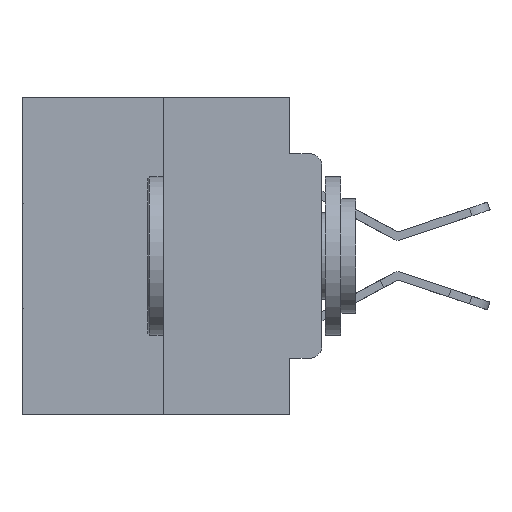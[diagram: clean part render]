
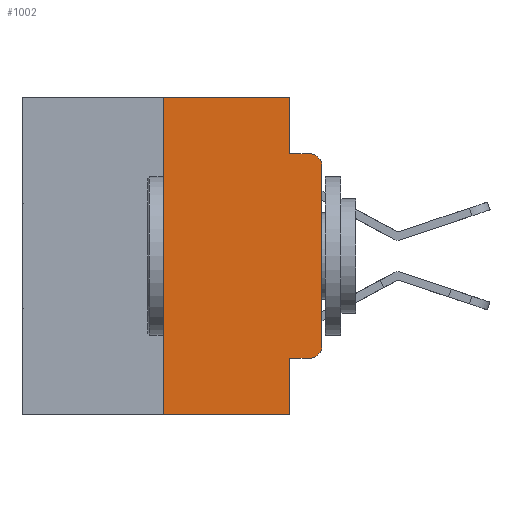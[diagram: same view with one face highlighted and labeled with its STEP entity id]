
A CAD part, left-side view. The second image highlights one B-rep face of the part: STEP entity #1002.
In plain terms, the highlighted planar face has unit normal (-1, 0, 0).
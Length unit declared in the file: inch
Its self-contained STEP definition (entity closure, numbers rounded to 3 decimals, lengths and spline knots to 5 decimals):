
#64 = CIRCLE ( 'NONE', #6986, 0.02 ) ;
#742 = DIRECTION ( 'NONE',  ( 0., -1., 0. ) ) ;
#959 = EDGE_CURVE ( 'NONE', #15801, #18309, #8363, .T. ) ;
#1002 = ADVANCED_FACE ( 'NONE', ( #3110 ), #13808, .F. ) ;
#1123 = DIRECTION ( 'NONE',  ( 0., 0., 1. ) ) ;
#1783 = CARTESIAN_POINT ( 'NONE',  ( 0., 0.473, 0. ) ) ;
#2193 = CARTESIAN_POINT ( 'NONE',  ( 0., 0.051, -0.4115 ) ) ;
#2379 = CIRCLE ( 'NONE', #25160, 0.02 ) ;
#3077 = ORIENTED_EDGE ( 'NONE', *, *, #23673, .F. ) ;
#3110 = FACE_OUTER_BOUND ( 'NONE', #18369, .T. ) ;
#3456 = LINE ( 'NONE', #24547, #14738 ) ;
#4176 = LINE ( 'NONE', #27578, #14776 ) ;
#4309 = AXIS2_PLACEMENT_3D ( 'NONE', #1783, #17391, #17080 ) ;
#4552 = VERTEX_POINT ( 'NONE', #12785 ) ;
#4573 = EDGE_CURVE ( 'NONE', #16203, #19289, #7102, .T. ) ;
#4838 = LINE ( 'NONE', #7823, #10851 ) ;
#6986 = AXIS2_PLACEMENT_3D ( 'NONE', #11329, #27059, #13607 ) ;
#7102 = LINE ( 'NONE', #12881, #24487 ) ;
#7797 = VECTOR ( 'NONE', #16236, 39.37008 ) ;
#7823 = CARTESIAN_POINT ( 'NONE',  ( 0., 0.051, 0. ) ) ;
#8363 = LINE ( 'NONE', #16173, #13659 ) ;
#8471 = VERTEX_POINT ( 'NONE', #2193 ) ;
#8494 = CARTESIAN_POINT ( 'NONE',  ( 0., 0.051, 0. ) ) ;
#8728 = ORIENTED_EDGE ( 'NONE', *, *, #24526, .F. ) ;
#9481 = VERTEX_POINT ( 'NONE', #17270 ) ;
#9647 = CARTESIAN_POINT ( 'NONE',  ( 0., 0.473, -0.5 ) ) ;
#10197 = CARTESIAN_POINT ( 'NONE',  ( 0., 0.25, -0.5 ) ) ;
#10491 = ORIENTED_EDGE ( 'NONE', *, *, #27255, .F. ) ;
#10586 = DIRECTION ( 'NONE',  ( 0., 0., 1. ) ) ;
#10818 = CARTESIAN_POINT ( 'NONE',  ( 0., 0.051, 0. ) ) ;
#10851 = VECTOR ( 'NONE', #12382, 39.37008 ) ;
#10988 = EDGE_CURVE ( 'NONE', #8471, #4552, #13813, .T. ) ;
#11183 = CARTESIAN_POINT ( 'NONE',  ( 0., 0., -0.1085 ) ) ;
#11329 = CARTESIAN_POINT ( 'NONE',  ( 0., 0.02, -0.3915 ) ) ;
#11498 = LINE ( 'NONE', #8494, #16125 ) ;
#11652 = VERTEX_POINT ( 'NONE', #25169 ) ;
#11654 = CARTESIAN_POINT ( 'NONE',  ( 0., 0.051, -0.4115 ) ) ;
#11881 = DIRECTION ( 'NONE',  ( 0., -1., 0. ) ) ;
#12382 = DIRECTION ( 'NONE',  ( 0., 0., -1. ) ) ;
#12596 = ORIENTED_EDGE ( 'NONE', *, *, #17511, .T. ) ;
#12601 = CARTESIAN_POINT ( 'NONE',  ( 0., 0.02, -0.1085 ) ) ;
#12785 = CARTESIAN_POINT ( 'NONE',  ( 0., 0.02, -0.4115 ) ) ;
#12881 = CARTESIAN_POINT ( 'NONE',  ( 0., 0., 0. ) ) ;
#13041 = DIRECTION ( 'NONE',  ( 0., 0., -1. ) ) ;
#13262 = EDGE_CURVE ( 'NONE', #19289, #26048, #2379, .T. ) ;
#13351 = ORIENTED_EDGE ( 'NONE', *, *, #13262, .T. ) ;
#13607 = DIRECTION ( 'NONE',  ( 0., 0., -1. ) ) ;
#13659 = VECTOR ( 'NONE', #1123, 39.37008 ) ;
#13808 = PLANE ( 'NONE',  #4309 ) ;
#13813 = LINE ( 'NONE', #11654, #7797 ) ;
#13824 = CARTESIAN_POINT ( 'NONE',  ( 0., 0., -0.3915 ) ) ;
#14233 = CARTESIAN_POINT ( 'NONE',  ( 0., 0.02, -0.0885 ) ) ;
#14548 = CARTESIAN_POINT ( 'NONE',  ( 0., 0.25, 0. ) ) ;
#14738 = VECTOR ( 'NONE', #26820, 39.37008 ) ;
#14776 = VECTOR ( 'NONE', #11881, 39.37008 ) ;
#14888 = DIRECTION ( 'NONE',  ( 0., 0., -1. ) ) ;
#15801 = VERTEX_POINT ( 'NONE', #10197 ) ;
#16125 = VECTOR ( 'NONE', #13041, 39.37008 ) ;
#16173 = CARTESIAN_POINT ( 'NONE',  ( 0., 0.25, 0. ) ) ;
#16203 = VERTEX_POINT ( 'NONE', #13824 ) ;
#16236 = DIRECTION ( 'NONE',  ( 0., -1., 0. ) ) ;
#17080 = DIRECTION ( 'NONE',  ( 0., 0., -1. ) ) ;
#17270 = CARTESIAN_POINT ( 'NONE',  ( 0., 0.051, -0.5 ) ) ;
#17391 = DIRECTION ( 'NONE',  ( 1., 0., 0. ) ) ;
#17511 = EDGE_CURVE ( 'NONE', #15801, #9481, #26097, .T. ) ;
#18309 = VERTEX_POINT ( 'NONE', #14548 ) ;
#18369 = EDGE_LOOP ( 'NONE', ( #18959, #13351, #25698, #8728, #10491, #28712, #12596, #3077, #18605, #27938 ) ) ;
#18605 = ORIENTED_EDGE ( 'NONE', *, *, #10988, .T. ) ;
#18756 = VECTOR ( 'NONE', #742, 39.37008 ) ;
#18959 = ORIENTED_EDGE ( 'NONE', *, *, #4573, .T. ) ;
#19289 = VERTEX_POINT ( 'NONE', #11183 ) ;
#23673 = EDGE_CURVE ( 'NONE', #8471, #9481, #4838, .T. ) ;
#24487 = VECTOR ( 'NONE', #10586, 39.37008 ) ;
#24526 = EDGE_CURVE ( 'NONE', #27991, #11652, #11498, .T. ) ;
#24547 = CARTESIAN_POINT ( 'NONE',  ( 0., 0.051, -0.0885 ) ) ;
#25160 = AXIS2_PLACEMENT_3D ( 'NONE', #12601, #28265, #14888 ) ;
#25169 = CARTESIAN_POINT ( 'NONE',  ( 0., 0.051, -0.0885 ) ) ;
#25698 = ORIENTED_EDGE ( 'NONE', *, *, #27659, .F. ) ;
#26048 = VERTEX_POINT ( 'NONE', #14233 ) ;
#26097 = LINE ( 'NONE', #9647, #18756 ) ;
#26473 = EDGE_CURVE ( 'NONE', #4552, #16203, #64, .T. ) ;
#26820 = DIRECTION ( 'NONE',  ( 0., -1., 0. ) ) ;
#27059 = DIRECTION ( 'NONE',  ( -1., 0., 0. ) ) ;
#27255 = EDGE_CURVE ( 'NONE', #18309, #27991, #4176, .T. ) ;
#27578 = CARTESIAN_POINT ( 'NONE',  ( 0., 0.473, 0. ) ) ;
#27659 = EDGE_CURVE ( 'NONE', #11652, #26048, #3456, .T. ) ;
#27938 = ORIENTED_EDGE ( 'NONE', *, *, #26473, .T. ) ;
#27991 = VERTEX_POINT ( 'NONE', #10818 ) ;
#28265 = DIRECTION ( 'NONE',  ( -1., 0., 0. ) ) ;
#28712 = ORIENTED_EDGE ( 'NONE', *, *, #959, .F. ) ;
